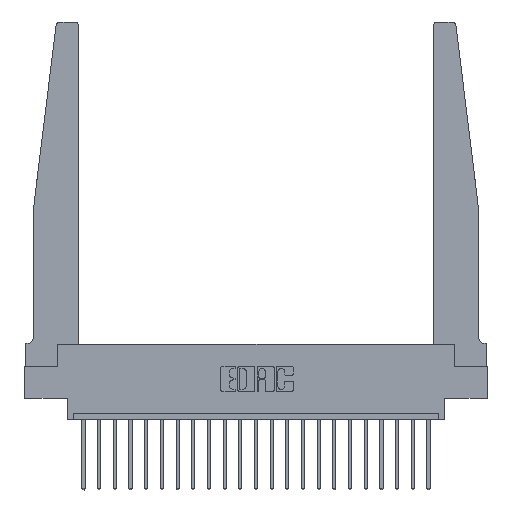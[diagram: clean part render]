
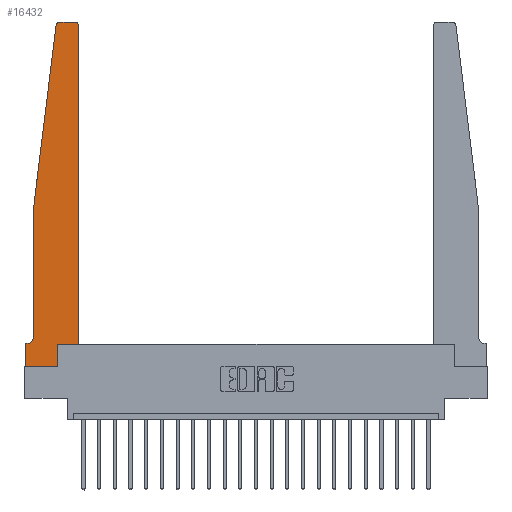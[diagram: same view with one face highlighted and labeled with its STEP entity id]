
A CAD part, top view. The second image highlights one B-rep face of the part: STEP entity #16432.
In plain terms, the highlighted planar face has unit normal (0, 0, 1).
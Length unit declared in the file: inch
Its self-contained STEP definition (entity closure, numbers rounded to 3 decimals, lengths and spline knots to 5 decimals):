
#153 = DIRECTION ( 'NONE',  ( 1., 0., 0. ) ) ;
#183 = VERTEX_POINT ( 'NONE', #7545 ) ;
#410 = EDGE_CURVE ( 'NONE', #16033, #13761, #17982, .T. ) ;
#462 = EDGE_CURVE ( 'NONE', #14239, #1780, #17732, .T. ) ;
#954 = VERTEX_POINT ( 'NONE', #1320 ) ;
#1101 = CARTESIAN_POINT ( 'NONE',  ( 0., 0., 0.37 ) ) ;
#1107 = CARTESIAN_POINT ( 'NONE',  ( 0.25, 2.75, 0.37 ) ) ;
#1320 = CARTESIAN_POINT ( 'NONE',  ( 0.065, 1.25, 0.37 ) ) ;
#1381 = VERTEX_POINT ( 'NONE', #7973 ) ;
#1589 = AXIS2_PLACEMENT_3D ( 'NONE', #5417, #17048, #8665 ) ;
#1780 = VERTEX_POINT ( 'NONE', #12517 ) ;
#1800 = VERTEX_POINT ( 'NONE', #17600 ) ;
#1931 = VECTOR ( 'NONE', #15216, 39.37008 ) ;
#2153 = EDGE_CURVE ( 'NONE', #15327, #16033, #20521, .T. ) ;
#2731 = CARTESIAN_POINT ( 'NONE',  ( 0.27653, 2.72, 0.37 ) ) ;
#2804 = DIRECTION ( 'NONE',  ( 0., 0., 1. ) ) ;
#3115 = ORIENTED_EDGE ( 'NONE', *, *, #4151, .T. ) ;
#3658 = ORIENTED_EDGE ( 'NONE', *, *, #7016, .T. ) ;
#4002 = CARTESIAN_POINT ( 'NONE',  ( 0.2605, 0.18, 0.37 ) ) ;
#4012 = ORIENTED_EDGE ( 'NONE', *, *, #21269, .T. ) ;
#4054 = EDGE_CURVE ( 'NONE', #13761, #16527, #14411, .T. ) ;
#4151 = EDGE_CURVE ( 'NONE', #1800, #1381, #16016, .T. ) ;
#4316 = AXIS2_PLACEMENT_3D ( 'NONE', #11197, #6294, #21234 ) ;
#4640 = DIRECTION ( 'NONE',  ( -1., 0., 0. ) ) ;
#4731 = DIRECTION ( 'NONE',  ( 1., 0., 0. ) ) ;
#4934 = DIRECTION ( 'NONE',  ( 0., 0., 1. ) ) ;
#5417 = CARTESIAN_POINT ( 'NONE',  ( 0., 0.1875, 0.37 ) ) ;
#5619 = VECTOR ( 'NONE', #9386, 39.37008 ) ;
#5714 = DIRECTION ( 'NONE',  ( 0., 1., 0. ) ) ;
#6170 = DIRECTION ( 'NONE',  ( 1., 0., 0. ) ) ;
#6294 = DIRECTION ( 'NONE',  ( 0., 0., -1. ) ) ;
#6332 = FACE_OUTER_BOUND ( 'NONE', #6523, .T. ) ;
#6523 = EDGE_LOOP ( 'NONE', ( #4012, #3115, #11017, #16306, #3658, #9642, #15450, #21591, #20808, #21681, #13859, #16198 ) ) ;
#6536 = VECTOR ( 'NONE', #18794, 39.37008 ) ;
#6636 = AXIS2_PLACEMENT_3D ( 'NONE', #15017, #4934, #153 ) ;
#6749 = EDGE_CURVE ( 'NONE', #1381, #954, #10118, .T. ) ;
#7016 = EDGE_CURVE ( 'NONE', #12916, #14239, #19585, .T. ) ;
#7128 = CARTESIAN_POINT ( 'NONE',  ( 0.425, 0.18, 0.37 ) ) ;
#7545 = CARTESIAN_POINT ( 'NONE',  ( 0.395, 2.75, 0.37 ) ) ;
#7637 = CARTESIAN_POINT ( 'NONE',  ( 0., 0., 0.37 ) ) ;
#7973 = CARTESIAN_POINT ( 'NONE',  ( 0.24675, 2.72367, 0.37 ) ) ;
#8162 = LINE ( 'NONE', #17434, #16587 ) ;
#8665 = DIRECTION ( 'NONE',  ( 1., 0., 0. ) ) ;
#8737 = VERTEX_POINT ( 'NONE', #14503 ) ;
#9386 = DIRECTION ( 'NONE',  ( -1., 0., 0. ) ) ;
#9642 = ORIENTED_EDGE ( 'NONE', *, *, #462, .T. ) ;
#10118 = LINE ( 'NONE', #10370, #1931 ) ;
#10288 = PLANE ( 'NONE',  #1589 ) ;
#10370 = CARTESIAN_POINT ( 'NONE',  ( 0.065, 1.25, 0.37 ) ) ;
#10463 = CIRCLE ( 'NONE', #6636, 0.03 ) ;
#10658 = DIRECTION ( 'NONE',  ( 0., -1., 0. ) ) ;
#11017 = ORIENTED_EDGE ( 'NONE', *, *, #6749, .T. ) ;
#11197 = CARTESIAN_POINT ( 'NONE',  ( 0.015, 0.2375, 0.37 ) ) ;
#11322 = EDGE_CURVE ( 'NONE', #16527, #8737, #15099, .T. ) ;
#11433 = VECTOR ( 'NONE', #12577, 39.37008 ) ;
#11911 = AXIS2_PLACEMENT_3D ( 'NONE', #2731, #2804, #4731 ) ;
#12017 = CARTESIAN_POINT ( 'NONE',  ( 0.065, 0.2375, 0.37 ) ) ;
#12517 = CARTESIAN_POINT ( 'NONE',  ( 0., 0.1875, 0.37 ) ) ;
#12568 = LINE ( 'NONE', #20324, #18104 ) ;
#12577 = DIRECTION ( 'NONE',  ( 0., 1., 0. ) ) ;
#12688 = CARTESIAN_POINT ( 'NONE',  ( 0.065, 0.1875, 0.37 ) ) ;
#12916 = VERTEX_POINT ( 'NONE', #12017 ) ;
#13642 = DIRECTION ( 'NONE',  ( 0., -1., 0. ) ) ;
#13761 = VERTEX_POINT ( 'NONE', #19172 ) ;
#13859 = ORIENTED_EDGE ( 'NONE', *, *, #11322, .T. ) ;
#14239 = VERTEX_POINT ( 'NONE', #18507 ) ;
#14411 = LINE ( 'NONE', #7128, #6536 ) ;
#14503 = CARTESIAN_POINT ( 'NONE',  ( 0.425, 2.72, 0.37 ) ) ;
#14558 = VECTOR ( 'NONE', #5714, 39.37008 ) ;
#15017 = CARTESIAN_POINT ( 'NONE',  ( 0.395, 2.72, 0.37 ) ) ;
#15099 = LINE ( 'NONE', #20926, #11433 ) ;
#15216 = DIRECTION ( 'NONE',  ( -0.122, -0.992, 0. ) ) ;
#15327 = VERTEX_POINT ( 'NONE', #1101 ) ;
#15448 = LINE ( 'NONE', #1107, #21693 ) ;
#15450 = ORIENTED_EDGE ( 'NONE', *, *, #19904, .T. ) ;
#16016 = CIRCLE ( 'NONE', #11911, 0.03 ) ;
#16033 = VERTEX_POINT ( 'NONE', #21061 ) ;
#16198 = ORIENTED_EDGE ( 'NONE', *, *, #20221, .T. ) ;
#16306 = ORIENTED_EDGE ( 'NONE', *, *, #19283, .T. ) ;
#16432 = ADVANCED_FACE ( 'NONE', ( #6332 ), #10288, .T. ) ;
#16527 = VERTEX_POINT ( 'NONE', #17553 ) ;
#16587 = VECTOR ( 'NONE', #10658, 39.37008 ) ;
#17048 = DIRECTION ( 'NONE',  ( 0., 0., 1. ) ) ;
#17434 = CARTESIAN_POINT ( 'NONE',  ( 0.065, 1.25, 0.37 ) ) ;
#17553 = CARTESIAN_POINT ( 'NONE',  ( 0.425, 0.18, 0.37 ) ) ;
#17600 = CARTESIAN_POINT ( 'NONE',  ( 0.27653, 2.75, 0.37 ) ) ;
#17732 = LINE ( 'NONE', #12688, #5619 ) ;
#17982 = LINE ( 'NONE', #4002, #14558 ) ;
#18104 = VECTOR ( 'NONE', #13642, 39.37008 ) ;
#18432 = VECTOR ( 'NONE', #6170, 39.37008 ) ;
#18507 = CARTESIAN_POINT ( 'NONE',  ( 0.015, 0.1875, 0.37 ) ) ;
#18794 = DIRECTION ( 'NONE',  ( 1., 0., 0. ) ) ;
#19172 = CARTESIAN_POINT ( 'NONE',  ( 0.2605, 0.18, 0.37 ) ) ;
#19283 = EDGE_CURVE ( 'NONE', #954, #12916, #8162, .T. ) ;
#19585 = CIRCLE ( 'NONE', #4316, 0.05 ) ;
#19904 = EDGE_CURVE ( 'NONE', #1780, #15327, #12568, .T. ) ;
#20221 = EDGE_CURVE ( 'NONE', #8737, #183, #10463, .T. ) ;
#20324 = CARTESIAN_POINT ( 'NONE',  ( 0., 0., 0.37 ) ) ;
#20521 = LINE ( 'NONE', #7637, #18432 ) ;
#20808 = ORIENTED_EDGE ( 'NONE', *, *, #410, .T. ) ;
#20926 = CARTESIAN_POINT ( 'NONE',  ( 0.425, 0.18, 0.37 ) ) ;
#21061 = CARTESIAN_POINT ( 'NONE',  ( 0.2605, 0., 0.37 ) ) ;
#21234 = DIRECTION ( 'NONE',  ( -1., 0., 0. ) ) ;
#21269 = EDGE_CURVE ( 'NONE', #183, #1800, #15448, .T. ) ;
#21591 = ORIENTED_EDGE ( 'NONE', *, *, #2153, .T. ) ;
#21681 = ORIENTED_EDGE ( 'NONE', *, *, #4054, .T. ) ;
#21693 = VECTOR ( 'NONE', #4640, 39.37008 ) ;
